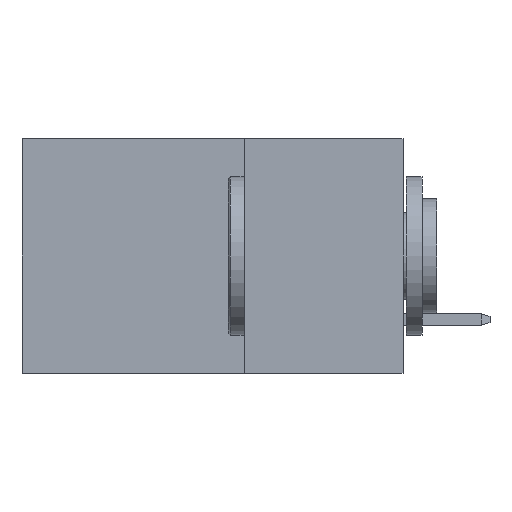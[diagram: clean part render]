
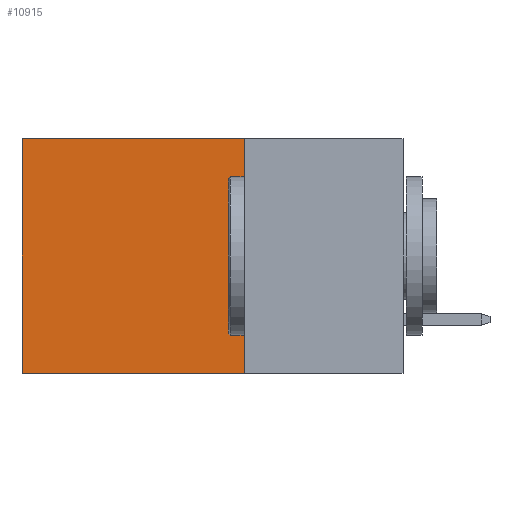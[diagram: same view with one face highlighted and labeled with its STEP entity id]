
A CAD part, left-side view. The second image highlights one B-rep face of the part: STEP entity #10915.
In plain terms, the highlighted planar face has unit normal (-1, 0, 0).
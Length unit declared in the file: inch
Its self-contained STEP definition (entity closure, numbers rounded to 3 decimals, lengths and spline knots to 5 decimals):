
#433 = DIRECTION ( 'NONE',  ( 0., 1., 0. ) ) ;
#739 = ORIENTED_EDGE ( 'NONE', *, *, #2218, .F. ) ;
#925 = ORIENTED_EDGE ( 'NONE', *, *, #12931, .T. ) ;
#1324 = LINE ( 'NONE', #4084, #14752 ) ;
#1875 = DIRECTION ( 'NONE',  ( 0., 1., 0. ) ) ;
#2023 = DIRECTION ( 'NONE',  ( 0., 0., -1. ) ) ;
#2118 = EDGE_CURVE ( 'NONE', #8644, #17209, #1324, .T. ) ;
#2142 = CARTESIAN_POINT ( 'NONE',  ( 0.2875, 0.25, 0. ) ) ;
#2218 = EDGE_CURVE ( 'NONE', #17209, #13727, #15241, .T. ) ;
#2854 = VECTOR ( 'NONE', #433, 39.37008 ) ;
#4084 = CARTESIAN_POINT ( 'NONE',  ( 0.2875, 0.25, 0. ) ) ;
#4557 = CARTESIAN_POINT ( 'NONE',  ( 0.2875, 0.25, 0. ) ) ;
#5844 = AXIS2_PLACEMENT_3D ( 'NONE', #10193, #7369, #2023 ) ;
#5955 = CARTESIAN_POINT ( 'NONE',  ( 0.2875, 0.25, -0.37 ) ) ;
#7369 = DIRECTION ( 'NONE',  ( 1., 0., 0. ) ) ;
#7521 = EDGE_CURVE ( 'NONE', #8644, #8837, #14033, .T. ) ;
#7626 = ORIENTED_EDGE ( 'NONE', *, *, #2118, .F. ) ;
#8644 = VERTEX_POINT ( 'NONE', #2142 ) ;
#8837 = VERTEX_POINT ( 'NONE', #11971 ) ;
#9110 = CARTESIAN_POINT ( 'NONE',  ( 0.2875, 0.6, 0. ) ) ;
#9495 = DIRECTION ( 'NONE',  ( 0., 0., -1. ) ) ;
#10193 = CARTESIAN_POINT ( 'NONE',  ( 0.2875, 0.25, 0. ) ) ;
#10915 = ADVANCED_FACE ( 'NONE', ( #14261 ), #16912, .F. ) ;
#11971 = CARTESIAN_POINT ( 'NONE',  ( 0.2875, 0.6, 0. ) ) ;
#12249 = VECTOR ( 'NONE', #1875, 39.37008 ) ;
#12327 = EDGE_LOOP ( 'NONE', ( #925, #739, #7626, #15365 ) ) ;
#12528 = CARTESIAN_POINT ( 'NONE',  ( 0.2875, 0.25, -0.37 ) ) ;
#12931 = EDGE_CURVE ( 'NONE', #8837, #13727, #17161, .T. ) ;
#13727 = VERTEX_POINT ( 'NONE', #13926 ) ;
#13926 = CARTESIAN_POINT ( 'NONE',  ( 0.2875, 0.6, -0.37 ) ) ;
#14033 = LINE ( 'NONE', #4557, #12249 ) ;
#14261 = FACE_OUTER_BOUND ( 'NONE', #12327, .T. ) ;
#14752 = VECTOR ( 'NONE', #9495, 39.37008 ) ;
#14810 = VECTOR ( 'NONE', #17251, 39.37008 ) ;
#15241 = LINE ( 'NONE', #5955, #2854 ) ;
#15365 = ORIENTED_EDGE ( 'NONE', *, *, #7521, .T. ) ;
#16912 = PLANE ( 'NONE',  #5844 ) ;
#17161 = LINE ( 'NONE', #9110, #14810 ) ;
#17209 = VERTEX_POINT ( 'NONE', #12528 ) ;
#17251 = DIRECTION ( 'NONE',  ( 0., 0., -1. ) ) ;
